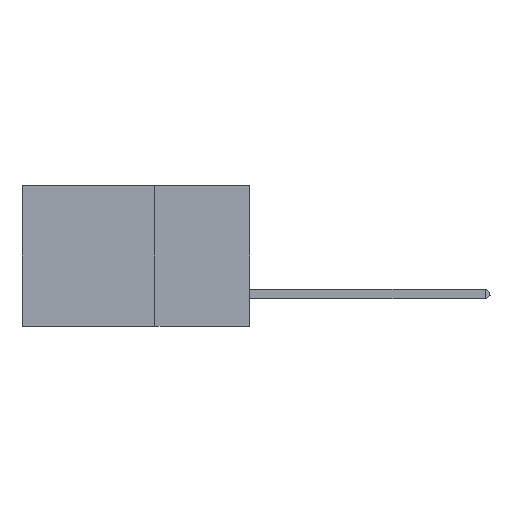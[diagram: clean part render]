
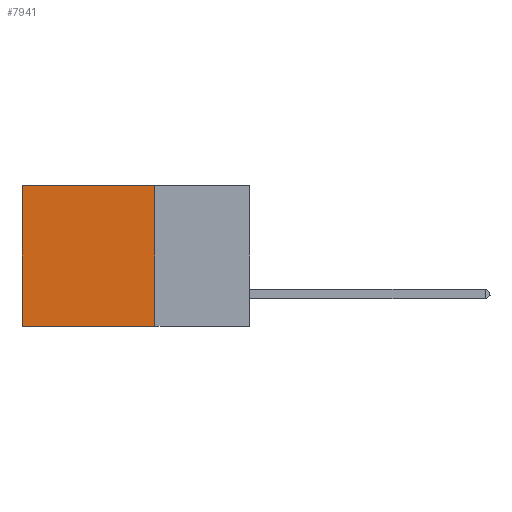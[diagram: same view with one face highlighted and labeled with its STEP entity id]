
A CAD part, left-side view. The second image highlights one B-rep face of the part: STEP entity #7941.
In plain terms, the highlighted planar face has unit normal (-1, 0, 0).
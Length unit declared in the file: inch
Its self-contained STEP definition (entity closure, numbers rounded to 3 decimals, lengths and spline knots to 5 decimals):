
#1816 = ORIENTED_EDGE ( 'NONE', *, *, #5122, .T. ) ;
#2599 = VERTEX_POINT ( 'NONE', #3605 ) ;
#3228 = DIRECTION ( 'NONE',  ( 0., 0., -1. ) ) ;
#3379 = DIRECTION ( 'NONE',  ( 0., 0., -1. ) ) ;
#3605 = CARTESIAN_POINT ( 'NONE',  ( 0.2875, 0.6, 0. ) ) ;
#3696 = CARTESIAN_POINT ( 'NONE',  ( 0.2875, 0.25, -0.37 ) ) ;
#4607 = LINE ( 'NONE', #7991, #15182 ) ;
#5122 = EDGE_CURVE ( 'NONE', #2599, #7898, #19624, .T. ) ;
#5188 = ORIENTED_EDGE ( 'NONE', *, *, #15219, .F. ) ;
#5281 = DIRECTION ( 'NONE',  ( 1., 0., 0. ) ) ;
#6654 = FACE_OUTER_BOUND ( 'NONE', #7152, .T. ) ;
#6662 = EDGE_CURVE ( 'NONE', #10402, #7898, #13075, .T. ) ;
#6753 = PLANE ( 'NONE',  #7178 ) ;
#7152 = EDGE_LOOP ( 'NONE', ( #1816, #19256, #5188, #10259 ) ) ;
#7178 = AXIS2_PLACEMENT_3D ( 'NONE', #14823, #5281, #3379 ) ;
#7889 = EDGE_CURVE ( 'NONE', #9630, #2599, #8235, .T. ) ;
#7898 = VERTEX_POINT ( 'NONE', #8251 ) ;
#7941 = ADVANCED_FACE ( 'NONE', ( #6654 ), #6753, .F. ) ;
#7991 = CARTESIAN_POINT ( 'NONE',  ( 0.2875, 0.25, 0. ) ) ;
#8235 = LINE ( 'NONE', #19374, #12585 ) ;
#8251 = CARTESIAN_POINT ( 'NONE',  ( 0.2875, 0.6, -0.37 ) ) ;
#8388 = CARTESIAN_POINT ( 'NONE',  ( 0.2875, 0.6, 0. ) ) ;
#8442 = DIRECTION ( 'NONE',  ( 0., 1., 0. ) ) ;
#8618 = CARTESIAN_POINT ( 'NONE',  ( 0.2875, 0.25, -0.37 ) ) ;
#9630 = VERTEX_POINT ( 'NONE', #14798 ) ;
#10095 = DIRECTION ( 'NONE',  ( 0., 1., 0. ) ) ;
#10259 = ORIENTED_EDGE ( 'NONE', *, *, #7889, .T. ) ;
#10402 = VERTEX_POINT ( 'NONE', #3696 ) ;
#12585 = VECTOR ( 'NONE', #8442, 39.37008 ) ;
#12965 = DIRECTION ( 'NONE',  ( 0., 0., -1. ) ) ;
#13075 = LINE ( 'NONE', #8618, #13963 ) ;
#13963 = VECTOR ( 'NONE', #10095, 39.37008 ) ;
#14599 = VECTOR ( 'NONE', #3228, 39.37008 ) ;
#14798 = CARTESIAN_POINT ( 'NONE',  ( 0.2875, 0.25, 0. ) ) ;
#14823 = CARTESIAN_POINT ( 'NONE',  ( 0.2875, 0.25, 0. ) ) ;
#15182 = VECTOR ( 'NONE', #12965, 39.37008 ) ;
#15219 = EDGE_CURVE ( 'NONE', #9630, #10402, #4607, .T. ) ;
#19256 = ORIENTED_EDGE ( 'NONE', *, *, #6662, .F. ) ;
#19374 = CARTESIAN_POINT ( 'NONE',  ( 0.2875, 0.25, 0. ) ) ;
#19624 = LINE ( 'NONE', #8388, #14599 ) ;
